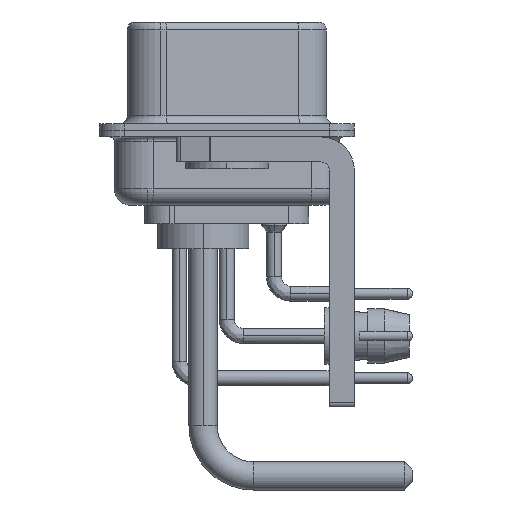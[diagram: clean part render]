
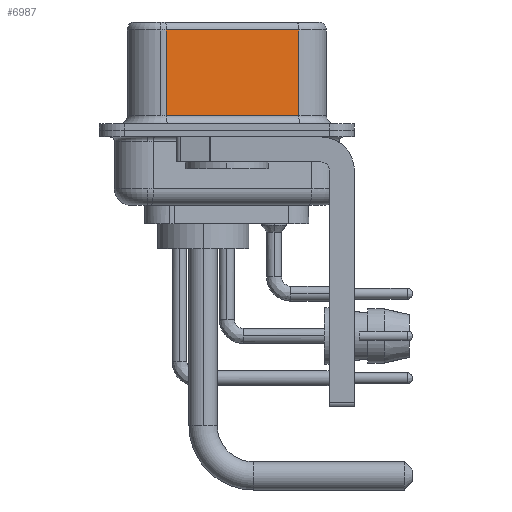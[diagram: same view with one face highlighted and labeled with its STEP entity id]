
A CAD part, left-side view. The second image highlights one B-rep face of the part: STEP entity #6987.
In plain terms, the highlighted planar face has unit normal (-0.985, -0.174, 0).
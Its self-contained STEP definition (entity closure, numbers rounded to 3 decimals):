
#162 = VECTOR ( 'NONE', #12912, 1000. ) ;
#676 = EDGE_CURVE ( 'NONE', #29744, #21530, #36019, .T. ) ;
#727 = LINE ( 'NONE', #12745, #17867 ) ;
#1374 = ORIENTED_EDGE ( 'NONE', *, *, #32217, .F. ) ;
#2324 = ORIENTED_EDGE ( 'NONE', *, *, #676, .T. ) ;
#2808 = DIRECTION ( 'NONE',  ( 0.985, 0.174, 0. ) ) ;
#4673 = VECTOR ( 'NONE', #34108, 1000. ) ;
#6987 = ADVANCED_FACE ( 'NONE', ( #8366 ), #16863, .F. ) ;
#8366 = FACE_OUTER_BOUND ( 'NONE', #9905, .T. ) ;
#8579 = CARTESIAN_POINT ( 'NONE',  ( 5.132, -4.322, 0.9 ) ) ;
#9152 = VECTOR ( 'NONE', #30420, 1000. ) ;
#9701 = CARTESIAN_POINT ( 'NONE',  ( 3.73, 3.628, 6.02 ) ) ;
#9905 = EDGE_LOOP ( 'NONE', ( #1374, #2324, #32771, #20886 ) ) ;
#11322 = DIRECTION ( 'NONE',  ( -0.174, 0.985, 0. ) ) ;
#12745 = CARTESIAN_POINT ( 'NONE',  ( 5.132, -4.322, 6.52 ) ) ;
#12912 = DIRECTION ( 'NONE',  ( 0., 0., -1. ) ) ;
#13022 = CARTESIAN_POINT ( 'NONE',  ( 5.132, -4.322, 0.9 ) ) ;
#13866 = EDGE_CURVE ( 'NONE', #17285, #17075, #19677, .T. ) ;
#16863 = PLANE ( 'NONE',  #24786 ) ;
#17075 = VERTEX_POINT ( 'NONE', #13022 ) ;
#17285 = VERTEX_POINT ( 'NONE', #36154 ) ;
#17867 = VECTOR ( 'NONE', #29384, 1000. ) ;
#19323 = EDGE_CURVE ( 'NONE', #21530, #17285, #33242, .T. ) ;
#19677 = LINE ( 'NONE', #8579, #4673 ) ;
#20886 = ORIENTED_EDGE ( 'NONE', *, *, #13866, .T. ) ;
#21530 = VERTEX_POINT ( 'NONE', #9701 ) ;
#24786 = AXIS2_PLACEMENT_3D ( 'NONE', #28131, #2808, #11322 ) ;
#28131 = CARTESIAN_POINT ( 'NONE',  ( 5.132, -4.322, 6.52 ) ) ;
#29384 = DIRECTION ( 'NONE',  ( 0., 0., -1. ) ) ;
#29744 = VERTEX_POINT ( 'NONE', #31494 ) ;
#30420 = DIRECTION ( 'NONE',  ( -0.174, 0.985, 0. ) ) ;
#31494 = CARTESIAN_POINT ( 'NONE',  ( 5.132, -4.322, 6.02 ) ) ;
#32217 = EDGE_CURVE ( 'NONE', #29744, #17075, #727, .T. ) ;
#32771 = ORIENTED_EDGE ( 'NONE', *, *, #19323, .T. ) ;
#33242 = LINE ( 'NONE', #35859, #162 ) ;
#33395 = CARTESIAN_POINT ( 'NONE',  ( 5.132, -4.322, 6.02 ) ) ;
#34108 = DIRECTION ( 'NONE',  ( 0.174, -0.985, 0. ) ) ;
#35859 = CARTESIAN_POINT ( 'NONE',  ( 3.73, 3.628, 6.52 ) ) ;
#36019 = LINE ( 'NONE', #33395, #9152 ) ;
#36154 = CARTESIAN_POINT ( 'NONE',  ( 3.73, 3.628, 0.9 ) ) ;
